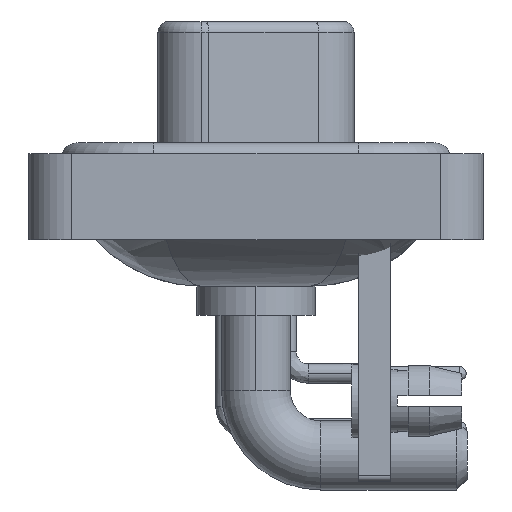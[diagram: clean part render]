
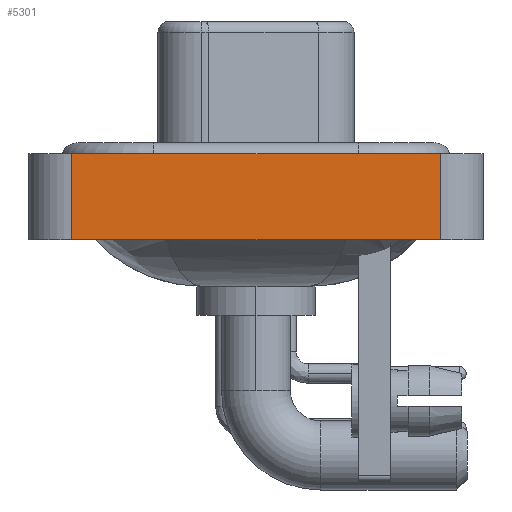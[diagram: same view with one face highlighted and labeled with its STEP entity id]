
A CAD part, left-side view. The second image highlights one B-rep face of the part: STEP entity #5301.
In plain terms, the highlighted planar face has unit normal (-1, 0, 0).
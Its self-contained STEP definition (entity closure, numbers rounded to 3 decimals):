
#2036 = EDGE_CURVE ( 'NONE', #17134, #27971, #16142, .T. ) ;
#2143 = CARTESIAN_POINT ( 'NONE',  ( -7.35, -8.55, 0.4 ) ) ;
#3265 = CARTESIAN_POINT ( 'NONE',  ( -7.35, 8.55, -3.6 ) ) ;
#3280 = DIRECTION ( 'NONE',  ( 0., -1., 0. ) ) ;
#3451 = VECTOR ( 'NONE', #3280, 1000. ) ;
#3731 = ORIENTED_EDGE ( 'NONE', *, *, #3963, .T. ) ;
#3963 = EDGE_CURVE ( 'NONE', #23458, #13634, #15367, .T. ) ;
#4389 = DIRECTION ( 'NONE',  ( 0., -1., 0. ) ) ;
#5105 = LINE ( 'NONE', #7838, #15115 ) ;
#5301 = ADVANCED_FACE ( 'NONE', ( #17381 ), #26145, .T. ) ;
#5435 = CARTESIAN_POINT ( 'NONE',  ( -7.35, -8.55, 0.4 ) ) ;
#5560 = EDGE_CURVE ( 'NONE', #23458, #17134, #5105, .T. ) ;
#6405 = CARTESIAN_POINT ( 'NONE',  ( -7.35, -8.55, -3.6 ) ) ;
#6579 = EDGE_LOOP ( 'NONE', ( #9926, #14604, #16901, #3731 ) ) ;
#7279 = CARTESIAN_POINT ( 'NONE',  ( -7.35, -8.55, -3.6 ) ) ;
#7838 = CARTESIAN_POINT ( 'NONE',  ( -7.35, 8.55, -3.6 ) ) ;
#8130 = EDGE_CURVE ( 'NONE', #13634, #27971, #27013, .T. ) ;
#9067 = VECTOR ( 'NONE', #4389, 1000. ) ;
#9926 = ORIENTED_EDGE ( 'NONE', *, *, #8130, .T. ) ;
#10097 = AXIS2_PLACEMENT_3D ( 'NONE', #6405, #15228, #24004 ) ;
#13634 = VERTEX_POINT ( 'NONE', #17462 ) ;
#14604 = ORIENTED_EDGE ( 'NONE', *, *, #2036, .F. ) ;
#15115 = VECTOR ( 'NONE', #21081, 1000. ) ;
#15228 = DIRECTION ( 'NONE',  ( -1., 0., 0. ) ) ;
#15367 = LINE ( 'NONE', #22552, #9067 ) ;
#16142 = LINE ( 'NONE', #5435, #3451 ) ;
#16901 = ORIENTED_EDGE ( 'NONE', *, *, #5560, .F. ) ;
#17134 = VERTEX_POINT ( 'NONE', #17573 ) ;
#17381 = FACE_OUTER_BOUND ( 'NONE', #6579, .T. ) ;
#17462 = CARTESIAN_POINT ( 'NONE',  ( -7.35, -8.55, -3.6 ) ) ;
#17573 = CARTESIAN_POINT ( 'NONE',  ( -7.35, 8.55, 0.4 ) ) ;
#21081 = DIRECTION ( 'NONE',  ( 0., 0., 1. ) ) ;
#21199 = VECTOR ( 'NONE', #24873, 1000. ) ;
#22552 = CARTESIAN_POINT ( 'NONE',  ( -7.35, -8.55, -3.6 ) ) ;
#23458 = VERTEX_POINT ( 'NONE', #3265 ) ;
#24004 = DIRECTION ( 'NONE',  ( 0., 0., 1. ) ) ;
#24873 = DIRECTION ( 'NONE',  ( 0., 0., 1. ) ) ;
#26145 = PLANE ( 'NONE',  #10097 ) ;
#27013 = LINE ( 'NONE', #7279, #21199 ) ;
#27971 = VERTEX_POINT ( 'NONE', #2143 ) ;
